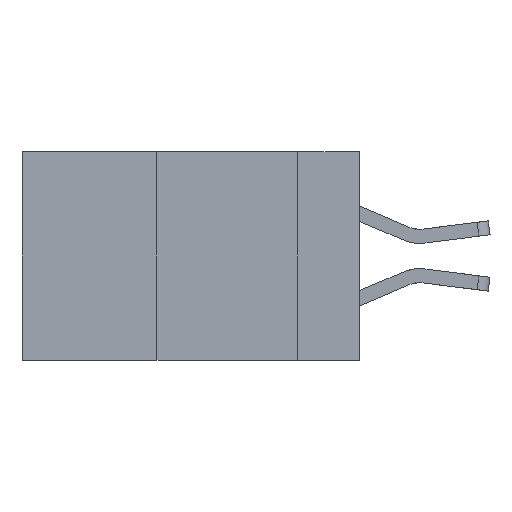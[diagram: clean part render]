
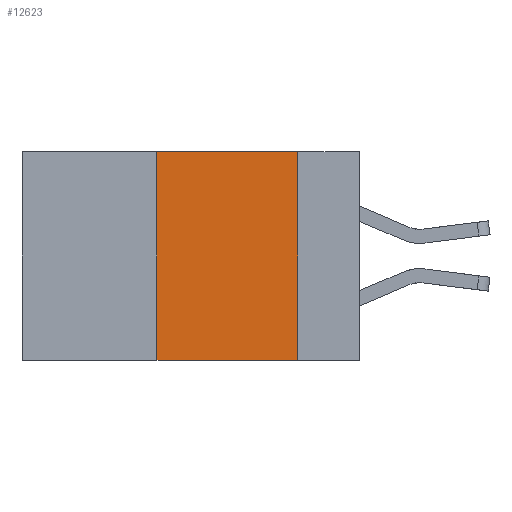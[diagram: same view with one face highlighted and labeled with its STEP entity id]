
A CAD part, left-side view. The second image highlights one B-rep face of the part: STEP entity #12623.
In plain terms, the highlighted planar face has unit normal (-1, 0, 0).
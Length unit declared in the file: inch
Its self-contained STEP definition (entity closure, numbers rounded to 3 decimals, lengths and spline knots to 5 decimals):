
#751 = PLANE ( 'NONE',  #12832 ) ;
#961 = ORIENTED_EDGE ( 'NONE', *, *, #3808, .F. ) ;
#2900 = VECTOR ( 'NONE', #5426, 39.37008 ) ;
#3151 = LINE ( 'NONE', #11186, #2900 ) ;
#3808 = EDGE_CURVE ( 'NONE', #12620, #7347, #14738, .T. ) ;
#4035 = VECTOR ( 'NONE', #9559, 39.37008 ) ;
#4108 = DIRECTION ( 'NONE',  ( 0., 0., -1. ) ) ;
#4233 = CARTESIAN_POINT ( 'NONE',  ( 0., 0.11, -0.37 ) ) ;
#4357 = CARTESIAN_POINT ( 'NONE',  ( 0., 0.11, 0. ) ) ;
#5426 = DIRECTION ( 'NONE',  ( 0., -1., 0. ) ) ;
#5462 = DIRECTION ( 'NONE',  ( 1., 0., 0. ) ) ;
#6057 = VECTOR ( 'NONE', #9543, 39.37008 ) ;
#6338 = VERTEX_POINT ( 'NONE', #13144 ) ;
#6829 = EDGE_CURVE ( 'NONE', #6338, #12620, #10697, .T. ) ;
#6860 = CARTESIAN_POINT ( 'NONE',  ( 0., 0.36, -0.37 ) ) ;
#7207 = ORIENTED_EDGE ( 'NONE', *, *, #13367, .T. ) ;
#7347 = VERTEX_POINT ( 'NONE', #4233 ) ;
#7359 = CARTESIAN_POINT ( 'NONE',  ( 0., 0.6, 0. ) ) ;
#7899 = VERTEX_POINT ( 'NONE', #6860 ) ;
#8195 = ORIENTED_EDGE ( 'NONE', *, *, #13978, .F. ) ;
#8326 = VECTOR ( 'NONE', #8970, 39.37008 ) ;
#8423 = EDGE_LOOP ( 'NONE', ( #961, #14820, #8195, #7207 ) ) ;
#8970 = DIRECTION ( 'NONE',  ( 0., 0., -1. ) ) ;
#9543 = DIRECTION ( 'NONE',  ( 0., 0., 1. ) ) ;
#9559 = DIRECTION ( 'NONE',  ( 0., -1., 0. ) ) ;
#10008 = FACE_OUTER_BOUND ( 'NONE', #8423, .T. ) ;
#10157 = CARTESIAN_POINT ( 'NONE',  ( 0., 0.6, 0. ) ) ;
#10697 = LINE ( 'NONE', #7359, #4035 ) ;
#10838 = LINE ( 'NONE', #13111, #6057 ) ;
#11186 = CARTESIAN_POINT ( 'NONE',  ( 0., 0.6, -0.37 ) ) ;
#12620 = VERTEX_POINT ( 'NONE', #14487 ) ;
#12623 = ADVANCED_FACE ( 'NONE', ( #10008 ), #751, .F. ) ;
#12832 = AXIS2_PLACEMENT_3D ( 'NONE', #10157, #5462, #4108 ) ;
#13111 = CARTESIAN_POINT ( 'NONE',  ( 0., 0.36, 0. ) ) ;
#13144 = CARTESIAN_POINT ( 'NONE',  ( 0., 0.36, 0. ) ) ;
#13367 = EDGE_CURVE ( 'NONE', #7899, #7347, #3151, .T. ) ;
#13978 = EDGE_CURVE ( 'NONE', #7899, #6338, #10838, .T. ) ;
#14487 = CARTESIAN_POINT ( 'NONE',  ( 0., 0.11, 0. ) ) ;
#14738 = LINE ( 'NONE', #4357, #8326 ) ;
#14820 = ORIENTED_EDGE ( 'NONE', *, *, #6829, .F. ) ;
